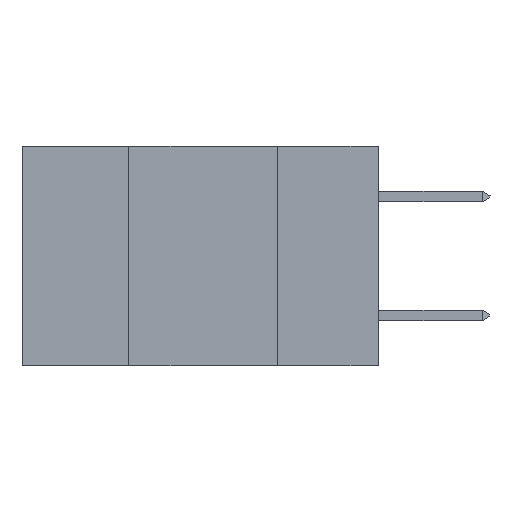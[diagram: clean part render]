
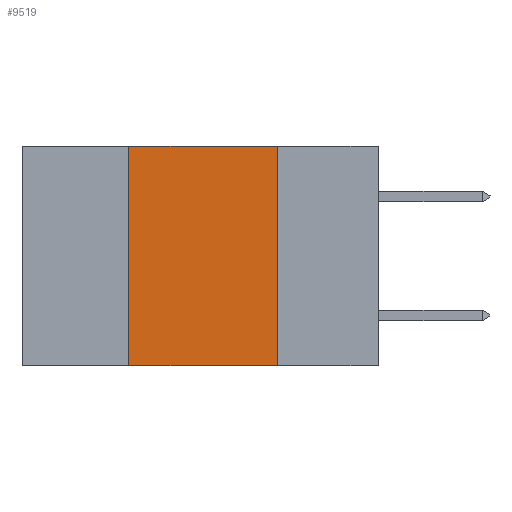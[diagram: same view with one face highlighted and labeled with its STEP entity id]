
A CAD part, left-side view. The second image highlights one B-rep face of the part: STEP entity #9519.
In plain terms, the highlighted planar face has unit normal (-1, 0, 0).
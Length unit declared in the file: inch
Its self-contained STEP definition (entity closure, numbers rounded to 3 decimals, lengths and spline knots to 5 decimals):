
#3 = CARTESIAN_POINT ( 'NONE',  ( 0., 0.17, 0. ) ) ;
#201 = CARTESIAN_POINT ( 'NONE',  ( 0., 0.6, 0. ) ) ;
#207 = ORIENTED_EDGE ( 'NONE', *, *, #1803, .F. ) ;
#265 = AXIS2_PLACEMENT_3D ( 'NONE', #201, #2001, #2854 ) ;
#574 = VECTOR ( 'NONE', #1549, 39.37008 ) ;
#785 = EDGE_CURVE ( 'NONE', #2757, #5493, #8119, .T. ) ;
#1366 = EDGE_LOOP ( 'NONE', ( #10637, #207, #4445, #8482 ) ) ;
#1478 = CARTESIAN_POINT ( 'NONE',  ( 0., 0.42, 0. ) ) ;
#1549 = DIRECTION ( 'NONE',  ( 0., 0., 1. ) ) ;
#1803 = EDGE_CURVE ( 'NONE', #5493, #9883, #7204, .T. ) ;
#2001 = DIRECTION ( 'NONE',  ( 1., 0., 0. ) ) ;
#2502 = CARTESIAN_POINT ( 'NONE',  ( 0., 0.6, 0. ) ) ;
#2641 = DIRECTION ( 'NONE',  ( 0., -1., 0. ) ) ;
#2757 = VERTEX_POINT ( 'NONE', #3247 ) ;
#2854 = DIRECTION ( 'NONE',  ( 0., 0., -1. ) ) ;
#3247 = CARTESIAN_POINT ( 'NONE',  ( 0., 0.42, -0.37 ) ) ;
#3893 = CARTESIAN_POINT ( 'NONE',  ( 0., 0.17, -0.37 ) ) ;
#3990 = VERTEX_POINT ( 'NONE', #7636 ) ;
#4445 = ORIENTED_EDGE ( 'NONE', *, *, #785, .F. ) ;
#5267 = DIRECTION ( 'NONE',  ( 0., -1., 0. ) ) ;
#5354 = CARTESIAN_POINT ( 'NONE',  ( 0., 0.42, -0.37 ) ) ;
#5493 = VERTEX_POINT ( 'NONE', #1478 ) ;
#5614 = VECTOR ( 'NONE', #2641, 39.37008 ) ;
#6185 = EDGE_CURVE ( 'NONE', #9883, #3990, #10300, .T. ) ;
#6342 = VECTOR ( 'NONE', #11204, 39.37008 ) ;
#6540 = FACE_OUTER_BOUND ( 'NONE', #1366, .T. ) ;
#7170 = CARTESIAN_POINT ( 'NONE',  ( 0., 0.6, -0.37 ) ) ;
#7204 = LINE ( 'NONE', #2502, #7329 ) ;
#7329 = VECTOR ( 'NONE', #5267, 39.37008 ) ;
#7636 = CARTESIAN_POINT ( 'NONE',  ( 0., 0.17, -0.37 ) ) ;
#8119 = LINE ( 'NONE', #5354, #574 ) ;
#8482 = ORIENTED_EDGE ( 'NONE', *, *, #10713, .T. ) ;
#9519 = ADVANCED_FACE ( 'NONE', ( #6540 ), #11071, .F. ) ;
#9883 = VERTEX_POINT ( 'NONE', #3 ) ;
#10300 = LINE ( 'NONE', #3893, #6342 ) ;
#10637 = ORIENTED_EDGE ( 'NONE', *, *, #6185, .F. ) ;
#10713 = EDGE_CURVE ( 'NONE', #2757, #3990, #10854, .T. ) ;
#10854 = LINE ( 'NONE', #7170, #5614 ) ;
#11071 = PLANE ( 'NONE',  #265 ) ;
#11204 = DIRECTION ( 'NONE',  ( 0., 0., -1. ) ) ;
